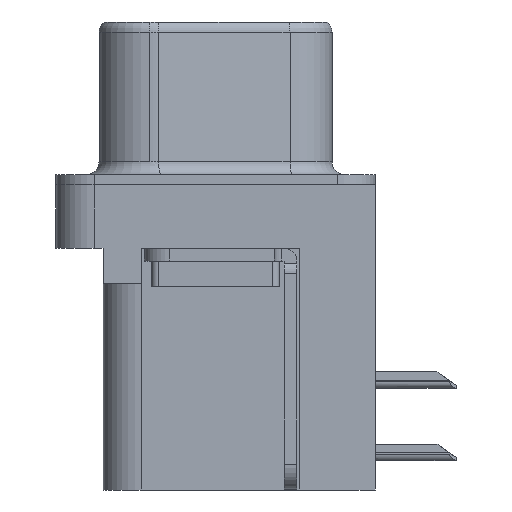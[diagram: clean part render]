
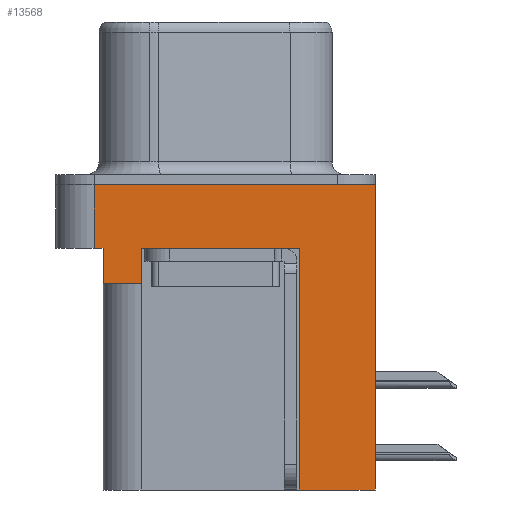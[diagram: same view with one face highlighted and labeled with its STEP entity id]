
A CAD part, left-side view. The second image highlights one B-rep face of the part: STEP entity #13568.
In plain terms, the highlighted planar face has unit normal (-1, 0, 0).
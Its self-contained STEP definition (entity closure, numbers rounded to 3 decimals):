
#744 = CARTESIAN_POINT ( 'NONE',  ( -3., -6.275, -2.5 ) ) ;
#919 = EDGE_CURVE ( 'NONE', #7186, #11647, #1058, .T. ) ;
#948 = CARTESIAN_POINT ( 'NONE',  ( -3., -6.275, -2.5 ) ) ;
#1058 = LINE ( 'NONE', #14328, #19185 ) ;
#1216 = DIRECTION ( 'NONE',  ( 0., -1., 0. ) ) ;
#1252 = LINE ( 'NONE', #1539, #1743 ) ;
#1370 = VERTEX_POINT ( 'NONE', #18577 ) ;
#1374 = EDGE_CURVE ( 'NONE', #9528, #6082, #8189, .T. ) ;
#1539 = CARTESIAN_POINT ( 'NONE',  ( -3., -6.275, 0. ) ) ;
#1568 = LINE ( 'NONE', #7474, #6732 ) ;
#1743 = VECTOR ( 'NONE', #7936, 1000. ) ;
#1994 = LINE ( 'NONE', #10817, #2271 ) ;
#2147 = LINE ( 'NONE', #18036, #8538 ) ;
#2271 = VECTOR ( 'NONE', #1216, 1000. ) ;
#2408 = VERTEX_POINT ( 'NONE', #19892 ) ;
#3049 = VECTOR ( 'NONE', #12708, 1000. ) ;
#3124 = AXIS2_PLACEMENT_3D ( 'NONE', #948, #8912, #19836 ) ;
#3382 = LINE ( 'NONE', #6102, #17822 ) ;
#4188 = DIRECTION ( 'NONE',  ( 0., 0., 1. ) ) ;
#4314 = ORIENTED_EDGE ( 'NONE', *, *, #919, .F. ) ;
#4368 = EDGE_CURVE ( 'NONE', #9526, #16715, #8053, .T. ) ;
#4730 = EDGE_CURVE ( 'NONE', #16715, #2408, #3382, .T. ) ;
#4883 = VERTEX_POINT ( 'NONE', #7904 ) ;
#5436 = VERTEX_POINT ( 'NONE', #16658 ) ;
#6082 = VERTEX_POINT ( 'NONE', #10704 ) ;
#6102 = CARTESIAN_POINT ( 'NONE',  ( -3., 4.425, -3.9 ) ) ;
#6732 = VECTOR ( 'NONE', #4188, 1000. ) ;
#6937 = LINE ( 'NONE', #744, #13303 ) ;
#7186 = VERTEX_POINT ( 'NONE', #9457 ) ;
#7358 = ORIENTED_EDGE ( 'NONE', *, *, #20149, .T. ) ;
#7474 = CARTESIAN_POINT ( 'NONE',  ( -3., 2.895, -3.9 ) ) ;
#7904 = CARTESIAN_POINT ( 'NONE',  ( -3., -6.275, 0. ) ) ;
#7936 = DIRECTION ( 'NONE',  ( 0., -1., 0. ) ) ;
#8053 = LINE ( 'NONE', #12854, #11969 ) ;
#8179 = CARTESIAN_POINT ( 'NONE',  ( -3., 4.425, -3.9 ) ) ;
#8189 = LINE ( 'NONE', #18703, #10849 ) ;
#8538 = VECTOR ( 'NONE', #14906, 1000. ) ;
#8619 = EDGE_CURVE ( 'NONE', #1370, #6082, #2147, .T. ) ;
#8784 = PLANE ( 'NONE',  #3124 ) ;
#8912 = DIRECTION ( 'NONE',  ( -1., 0., 0. ) ) ;
#9457 = CARTESIAN_POINT ( 'NONE',  ( -3., 4.775, -2.5 ) ) ;
#9526 = VERTEX_POINT ( 'NONE', #17729 ) ;
#9528 = VERTEX_POINT ( 'NONE', #17465 ) ;
#10006 = DIRECTION ( 'NONE',  ( 0., 0., 1. ) ) ;
#10423 = EDGE_CURVE ( 'NONE', #11647, #4883, #1252, .T. ) ;
#10633 = DIRECTION ( 'NONE',  ( 0., 0., 1. ) ) ;
#10634 = ORIENTED_EDGE ( 'NONE', *, *, #19477, .T. ) ;
#10648 = ORIENTED_EDGE ( 'NONE', *, *, #8619, .F. ) ;
#10704 = CARTESIAN_POINT ( 'NONE',  ( -3., -3.295, -2.5 ) ) ;
#10817 = CARTESIAN_POINT ( 'NONE',  ( -3., -6.275, -2.5 ) ) ;
#10849 = VECTOR ( 'NONE', #17009, 1000. ) ;
#11014 = CARTESIAN_POINT ( 'NONE',  ( -3., 4.775, 0. ) ) ;
#11647 = VERTEX_POINT ( 'NONE', #11014 ) ;
#11969 = VECTOR ( 'NONE', #12779, 1000. ) ;
#12137 = ORIENTED_EDGE ( 'NONE', *, *, #18330, .T. ) ;
#12708 = DIRECTION ( 'NONE',  ( 0., 1., 0. ) ) ;
#12779 = DIRECTION ( 'NONE',  ( 0., 1., 0. ) ) ;
#12808 = DIRECTION ( 'NONE',  ( 0., 0., 1. ) ) ;
#12854 = CARTESIAN_POINT ( 'NONE',  ( -3., 4.425, -3.9 ) ) ;
#12872 = LINE ( 'NONE', #19246, #3049 ) ;
#12976 = FACE_OUTER_BOUND ( 'NONE', #17772, .T. ) ;
#13303 = VECTOR ( 'NONE', #10006, 1000. ) ;
#13568 = ADVANCED_FACE ( 'NONE', ( #12976 ), #8784, .T. ) ;
#14328 = CARTESIAN_POINT ( 'NONE',  ( -3., 4.775, -2.5 ) ) ;
#14391 = EDGE_CURVE ( 'NONE', #5436, #1370, #12872, .T. ) ;
#14906 = DIRECTION ( 'NONE',  ( 0., 0., 1. ) ) ;
#15196 = ORIENTED_EDGE ( 'NONE', *, *, #4730, .F. ) ;
#16658 = CARTESIAN_POINT ( 'NONE',  ( -3., -6.275, -12. ) ) ;
#16715 = VERTEX_POINT ( 'NONE', #8179 ) ;
#17009 = DIRECTION ( 'NONE',  ( 0., -1., 0. ) ) ;
#17465 = CARTESIAN_POINT ( 'NONE',  ( -3., 2.895, -2.5 ) ) ;
#17550 = ORIENTED_EDGE ( 'NONE', *, *, #14391, .F. ) ;
#17729 = CARTESIAN_POINT ( 'NONE',  ( -3., 2.895, -3.9 ) ) ;
#17772 = EDGE_LOOP ( 'NONE', ( #18587, #4314, #7358, #15196, #18320, #12137, #19518, #10648, #17550, #10634 ) ) ;
#17822 = VECTOR ( 'NONE', #10633, 1000. ) ;
#18036 = CARTESIAN_POINT ( 'NONE',  ( -3., -3.295, -12. ) ) ;
#18320 = ORIENTED_EDGE ( 'NONE', *, *, #4368, .F. ) ;
#18330 = EDGE_CURVE ( 'NONE', #9526, #9528, #1568, .T. ) ;
#18577 = CARTESIAN_POINT ( 'NONE',  ( -3., -3.295, -12. ) ) ;
#18587 = ORIENTED_EDGE ( 'NONE', *, *, #10423, .F. ) ;
#18703 = CARTESIAN_POINT ( 'NONE',  ( -3., -6.275, -2.5 ) ) ;
#19185 = VECTOR ( 'NONE', #12808, 1000. ) ;
#19246 = CARTESIAN_POINT ( 'NONE',  ( -3., -3.295, -12. ) ) ;
#19477 = EDGE_CURVE ( 'NONE', #5436, #4883, #6937, .T. ) ;
#19518 = ORIENTED_EDGE ( 'NONE', *, *, #1374, .T. ) ;
#19836 = DIRECTION ( 'NONE',  ( 0., 0., 1. ) ) ;
#19892 = CARTESIAN_POINT ( 'NONE',  ( -3., 4.425, -2.5 ) ) ;
#20149 = EDGE_CURVE ( 'NONE', #7186, #2408, #1994, .T. ) ;
